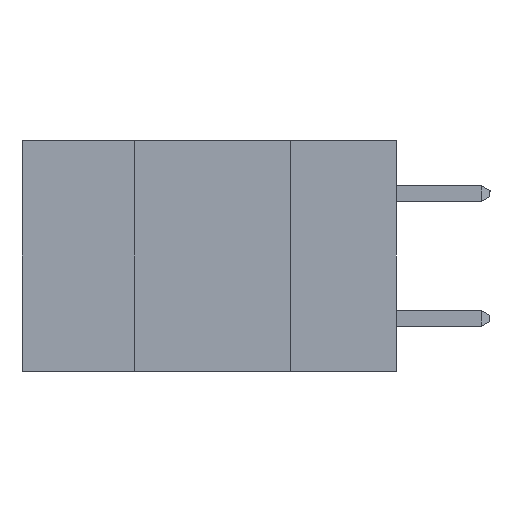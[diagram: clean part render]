
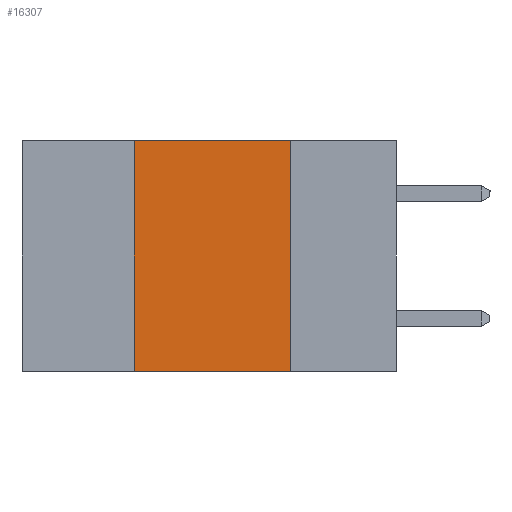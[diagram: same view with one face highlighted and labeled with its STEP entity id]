
A CAD part, left-side view. The second image highlights one B-rep face of the part: STEP entity #16307.
In plain terms, the highlighted planar face has unit normal (-1, 0, 0).
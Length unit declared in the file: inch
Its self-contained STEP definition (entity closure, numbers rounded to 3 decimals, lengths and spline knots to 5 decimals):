
#99 = LINE ( 'NONE', #17669, #8457 ) ;
#898 = DIRECTION ( 'NONE',  ( 0., 0., -1. ) ) ;
#1106 = LINE ( 'NONE', #8561, #19767 ) ;
#1458 = EDGE_CURVE ( 'NONE', #2290, #6559, #99, .T. ) ;
#1775 = CARTESIAN_POINT ( 'NONE',  ( 0., 0.17, 0. ) ) ;
#2290 = VERTEX_POINT ( 'NONE', #4806 ) ;
#2427 = CARTESIAN_POINT ( 'NONE',  ( 0., 0.6, 0. ) ) ;
#2500 = ORIENTED_EDGE ( 'NONE', *, *, #1458, .T. ) ;
#2531 = FACE_OUTER_BOUND ( 'NONE', #12025, .T. ) ;
#2876 = ORIENTED_EDGE ( 'NONE', *, *, #19620, .F. ) ;
#2944 = DIRECTION ( 'NONE',  ( 0., 0., 1. ) ) ;
#3152 = VERTEX_POINT ( 'NONE', #12970 ) ;
#3476 = ORIENTED_EDGE ( 'NONE', *, *, #10659, .F. ) ;
#4511 = VECTOR ( 'NONE', #2944, 39.37008 ) ;
#4806 = CARTESIAN_POINT ( 'NONE',  ( 0., 0.42, -0.37 ) ) ;
#5832 = VECTOR ( 'NONE', #11087, 39.37008 ) ;
#6559 = VERTEX_POINT ( 'NONE', #13618 ) ;
#7596 = LINE ( 'NONE', #17185, #4511 ) ;
#8056 = VERTEX_POINT ( 'NONE', #1775 ) ;
#8457 = VECTOR ( 'NONE', #11417, 39.37008 ) ;
#8561 = CARTESIAN_POINT ( 'NONE',  ( 0., 0.17, -0.37 ) ) ;
#8725 = DIRECTION ( 'NONE',  ( 1., 0., 0. ) ) ;
#10659 = EDGE_CURVE ( 'NONE', #3152, #8056, #11303, .T. ) ;
#11087 = DIRECTION ( 'NONE',  ( 0., -1., 0. ) ) ;
#11303 = LINE ( 'NONE', #17440, #5832 ) ;
#11417 = DIRECTION ( 'NONE',  ( 0., -1., 0. ) ) ;
#11791 = PLANE ( 'NONE',  #14701 ) ;
#12025 = EDGE_LOOP ( 'NONE', ( #19518, #3476, #2876, #2500 ) ) ;
#12970 = CARTESIAN_POINT ( 'NONE',  ( 0., 0.42, 0. ) ) ;
#13618 = CARTESIAN_POINT ( 'NONE',  ( 0., 0.17, -0.37 ) ) ;
#14416 = EDGE_CURVE ( 'NONE', #8056, #6559, #1106, .T. ) ;
#14701 = AXIS2_PLACEMENT_3D ( 'NONE', #2427, #8725, #18135 ) ;
#16307 = ADVANCED_FACE ( 'NONE', ( #2531 ), #11791, .F. ) ;
#17185 = CARTESIAN_POINT ( 'NONE',  ( 0., 0.42, -0.37 ) ) ;
#17440 = CARTESIAN_POINT ( 'NONE',  ( 0., 0.6, 0. ) ) ;
#17669 = CARTESIAN_POINT ( 'NONE',  ( 0., 0.6, -0.37 ) ) ;
#18135 = DIRECTION ( 'NONE',  ( 0., 0., -1. ) ) ;
#19518 = ORIENTED_EDGE ( 'NONE', *, *, #14416, .F. ) ;
#19620 = EDGE_CURVE ( 'NONE', #2290, #3152, #7596, .T. ) ;
#19767 = VECTOR ( 'NONE', #898, 39.37008 ) ;
